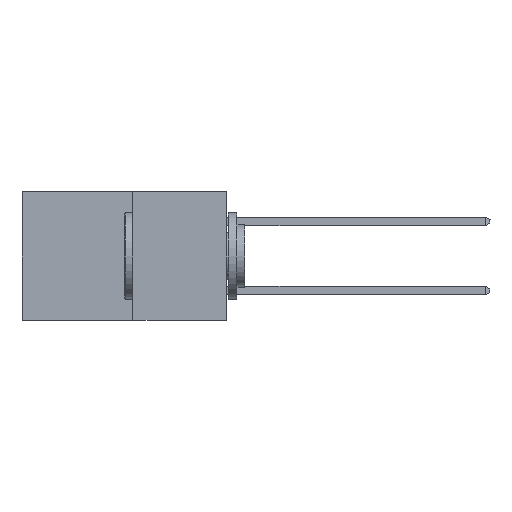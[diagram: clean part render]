
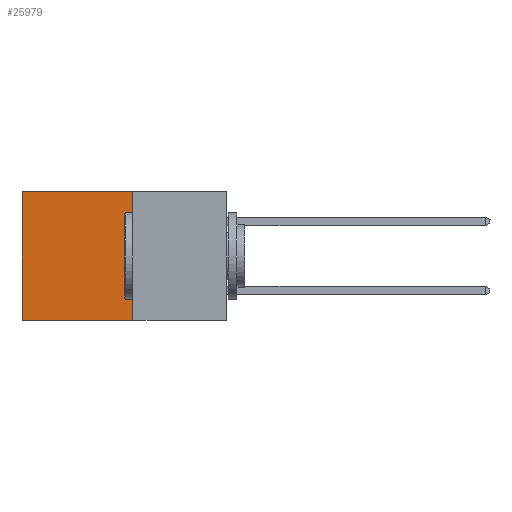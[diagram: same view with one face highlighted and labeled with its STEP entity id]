
A CAD part, left-side view. The second image highlights one B-rep face of the part: STEP entity #25979.
In plain terms, the highlighted planar face has unit normal (-1, 0, 0).
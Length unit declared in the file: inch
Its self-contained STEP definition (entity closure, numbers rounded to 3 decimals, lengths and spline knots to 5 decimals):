
#118 = ORIENTED_EDGE ( 'NONE', *, *, #31298, .T. ) ;
#767 = VERTEX_POINT ( 'NONE', #4515 ) ;
#950 = ORIENTED_EDGE ( 'NONE', *, *, #10287, .F. ) ;
#1804 = VECTOR ( 'NONE', #13232, 39.37008 ) ;
#2959 = LINE ( 'NONE', #18627, #30964 ) ;
#4515 = CARTESIAN_POINT ( 'NONE',  ( 0.277, 0.59, 0. ) ) ;
#7672 = CARTESIAN_POINT ( 'NONE',  ( 0.277, 0.27, -0.37 ) ) ;
#7958 = DIRECTION ( 'NONE',  ( 0., 1., 0. ) ) ;
#8003 = CARTESIAN_POINT ( 'NONE',  ( 0.277, 0.27, -0.37 ) ) ;
#9035 = LINE ( 'NONE', #10499, #1804 ) ;
#10287 = EDGE_CURVE ( 'NONE', #19558, #18882, #26904, .T. ) ;
#10499 = CARTESIAN_POINT ( 'NONE',  ( 0.277, 0.27, -0.37 ) ) ;
#10737 = DIRECTION ( 'NONE',  ( 1., 0., 0. ) ) ;
#10850 = LINE ( 'NONE', #16038, #24442 ) ;
#13232 = DIRECTION ( 'NONE',  ( 0., 1., 0. ) ) ;
#15729 = CARTESIAN_POINT ( 'NONE',  ( 0.277, 0.59, -0.37 ) ) ;
#16038 = CARTESIAN_POINT ( 'NONE',  ( 0.277, 0.27, 0. ) ) ;
#18219 = VERTEX_POINT ( 'NONE', #15729 ) ;
#18627 = CARTESIAN_POINT ( 'NONE',  ( 0.277, 0.59, -0.37 ) ) ;
#18748 = DIRECTION ( 'NONE',  ( 0., 0., -1. ) ) ;
#18882 = VERTEX_POINT ( 'NONE', #35074 ) ;
#19558 = VERTEX_POINT ( 'NONE', #29379 ) ;
#20917 = AXIS2_PLACEMENT_3D ( 'NONE', #8003, #10737, #29685 ) ;
#21669 = ORIENTED_EDGE ( 'NONE', *, *, #32636, .F. ) ;
#23116 = ORIENTED_EDGE ( 'NONE', *, *, #27510, .T. ) ;
#24442 = VECTOR ( 'NONE', #7958, 39.37008 ) ;
#25979 = ADVANCED_FACE ( 'NONE', ( #34326 ), #26982, .F. ) ;
#26649 = DIRECTION ( 'NONE',  ( 0., 0., -1. ) ) ;
#26904 = LINE ( 'NONE', #7672, #31501 ) ;
#26982 = PLANE ( 'NONE',  #20917 ) ;
#27510 = EDGE_CURVE ( 'NONE', #767, #18219, #2959, .T. ) ;
#29379 = CARTESIAN_POINT ( 'NONE',  ( 0.277, 0.27, 0. ) ) ;
#29685 = DIRECTION ( 'NONE',  ( 0., 0., -1. ) ) ;
#30029 = EDGE_LOOP ( 'NONE', ( #23116, #21669, #950, #118 ) ) ;
#30964 = VECTOR ( 'NONE', #18748, 39.37008 ) ;
#31298 = EDGE_CURVE ( 'NONE', #19558, #767, #10850, .T. ) ;
#31501 = VECTOR ( 'NONE', #26649, 39.37008 ) ;
#32636 = EDGE_CURVE ( 'NONE', #18882, #18219, #9035, .T. ) ;
#34326 = FACE_OUTER_BOUND ( 'NONE', #30029, .T. ) ;
#35074 = CARTESIAN_POINT ( 'NONE',  ( 0.277, 0.27, -0.37 ) ) ;
